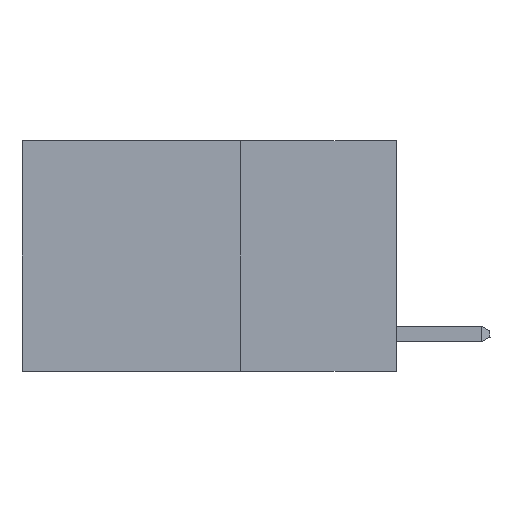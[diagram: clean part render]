
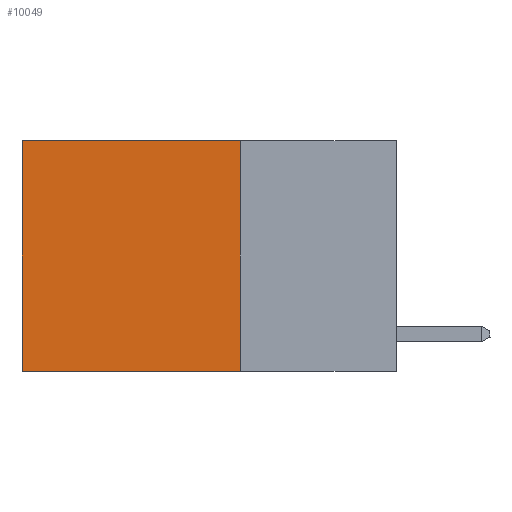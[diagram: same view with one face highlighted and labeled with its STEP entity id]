
A CAD part, left-side view. The second image highlights one B-rep face of the part: STEP entity #10049.
In plain terms, the highlighted planar face has unit normal (-1, 0, 0).
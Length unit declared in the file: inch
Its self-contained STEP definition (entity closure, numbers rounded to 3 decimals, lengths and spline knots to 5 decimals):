
#40 = VERTEX_POINT ( 'NONE', #3521 ) ;
#132 = CARTESIAN_POINT ( 'NONE',  ( 0.2625, 0.25, 0. ) ) ;
#1859 = EDGE_CURVE ( 'NONE', #9329, #5861, #6884, .T. ) ;
#2265 = DIRECTION ( 'NONE',  ( 0., 1., 0. ) ) ;
#3521 = CARTESIAN_POINT ( 'NONE',  ( 0.2625, 0.6, -0.37 ) ) ;
#3579 = ORIENTED_EDGE ( 'NONE', *, *, #1859, .T. ) ;
#3841 = LINE ( 'NONE', #10613, #11151 ) ;
#4008 = EDGE_CURVE ( 'NONE', #5861, #40, #7085, .T. ) ;
#4327 = VECTOR ( 'NONE', #2265, 39.37008 ) ;
#4882 = DIRECTION ( 'NONE',  ( 0., 1., 0. ) ) ;
#5095 = CARTESIAN_POINT ( 'NONE',  ( 0.2625, 0.25, 0. ) ) ;
#5660 = CARTESIAN_POINT ( 'NONE',  ( 0.2625, 0.6, 0. ) ) ;
#5701 = VECTOR ( 'NONE', #12038, 39.37008 ) ;
#5861 = VERTEX_POINT ( 'NONE', #6173 ) ;
#5982 = ORIENTED_EDGE ( 'NONE', *, *, #4008, .T. ) ;
#6029 = EDGE_CURVE ( 'NONE', #9329, #6489, #10782, .T. ) ;
#6066 = DIRECTION ( 'NONE',  ( 0., 0., -1. ) ) ;
#6173 = CARTESIAN_POINT ( 'NONE',  ( 0.2625, 0.6, 0. ) ) ;
#6489 = VERTEX_POINT ( 'NONE', #11137 ) ;
#6636 = DIRECTION ( 'NONE',  ( 0., 0., -1. ) ) ;
#6801 = VECTOR ( 'NONE', #6636, 39.37008 ) ;
#6884 = LINE ( 'NONE', #8198, #4327 ) ;
#7085 = LINE ( 'NONE', #5660, #6801 ) ;
#8198 = CARTESIAN_POINT ( 'NONE',  ( 0.2625, 0.25, 0. ) ) ;
#8974 = EDGE_CURVE ( 'NONE', #6489, #40, #3841, .T. ) ;
#9329 = VERTEX_POINT ( 'NONE', #132 ) ;
#9661 = FACE_OUTER_BOUND ( 'NONE', #11504, .T. ) ;
#9785 = ORIENTED_EDGE ( 'NONE', *, *, #6029, .F. ) ;
#10049 = ADVANCED_FACE ( 'NONE', ( #9661 ), #10825, .F. ) ;
#10148 = CARTESIAN_POINT ( 'NONE',  ( 0.2625, 0.25, 0. ) ) ;
#10613 = CARTESIAN_POINT ( 'NONE',  ( 0.2625, 0.25, -0.37 ) ) ;
#10782 = LINE ( 'NONE', #10148, #5701 ) ;
#10825 = PLANE ( 'NONE',  #11717 ) ;
#11137 = CARTESIAN_POINT ( 'NONE',  ( 0.2625, 0.25, -0.37 ) ) ;
#11151 = VECTOR ( 'NONE', #4882, 39.37008 ) ;
#11504 = EDGE_LOOP ( 'NONE', ( #5982, #11904, #9785, #3579 ) ) ;
#11717 = AXIS2_PLACEMENT_3D ( 'NONE', #5095, #11735, #6066 ) ;
#11735 = DIRECTION ( 'NONE',  ( 1., 0., 0. ) ) ;
#11904 = ORIENTED_EDGE ( 'NONE', *, *, #8974, .F. ) ;
#12038 = DIRECTION ( 'NONE',  ( 0., 0., -1. ) ) ;
